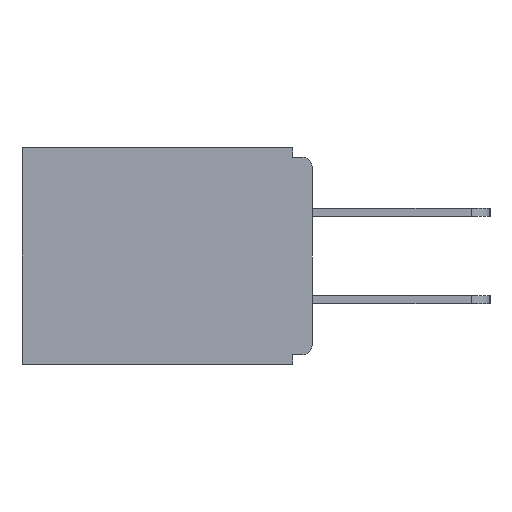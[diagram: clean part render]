
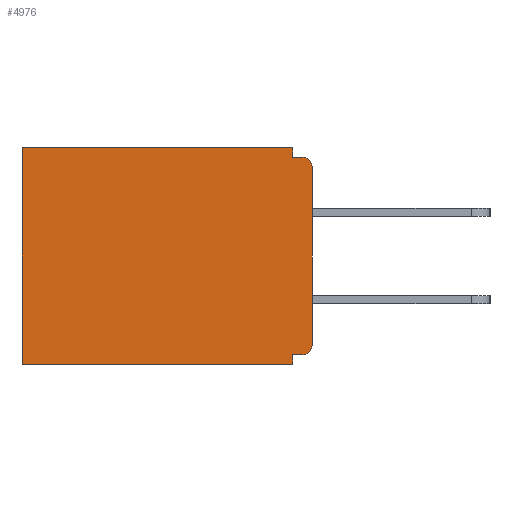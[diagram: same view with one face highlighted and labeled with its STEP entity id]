
A CAD part, left-side view. The second image highlights one B-rep face of the part: STEP entity #4976.
In plain terms, the highlighted planar face has unit normal (-1, 0, 0).
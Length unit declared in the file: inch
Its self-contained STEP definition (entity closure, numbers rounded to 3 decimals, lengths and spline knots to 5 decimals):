
#96 = CARTESIAN_POINT ( 'NONE',  ( 0.298, 0.46, 0. ) ) ;
#584 = ORIENTED_EDGE ( 'NONE', *, *, #10309, .F. ) ;
#746 = VECTOR ( 'NONE', #6360, 39.37008 ) ;
#1071 = CARTESIAN_POINT ( 'NONE',  ( 0.298, 0.031, -0.343 ) ) ;
#1100 = VERTEX_POINT ( 'NONE', #13510 ) ;
#1137 = VECTOR ( 'NONE', #1283, 39.37008 ) ;
#1283 = DIRECTION ( 'NONE',  ( 0., 0., -1. ) ) ;
#1432 = CARTESIAN_POINT ( 'NONE',  ( 0.298, 0., 0. ) ) ;
#1663 = CARTESIAN_POINT ( 'NONE',  ( 0.298, 0., -0.03 ) ) ;
#1769 = ORIENTED_EDGE ( 'NONE', *, *, #7219, .F. ) ;
#2150 = VECTOR ( 'NONE', #5401, 39.37008 ) ;
#2573 = ORIENTED_EDGE ( 'NONE', *, *, #8104, .T. ) ;
#2772 = DIRECTION ( 'NONE',  ( 1., 0., 0. ) ) ;
#2856 = LINE ( 'NONE', #5143, #14362 ) ;
#2864 = VERTEX_POINT ( 'NONE', #1663 ) ;
#2973 = DIRECTION ( 'NONE',  ( 0., 0., -1. ) ) ;
#3009 = DIRECTION ( 'NONE',  ( -1., 0., 0. ) ) ;
#3091 = DIRECTION ( 'NONE',  ( 0., 0., -1. ) ) ;
#3565 = CARTESIAN_POINT ( 'NONE',  ( 0.298, 0.46, -0.343 ) ) ;
#3988 = VECTOR ( 'NONE', #12578, 39.37008 ) ;
#4116 = CARTESIAN_POINT ( 'NONE',  ( 0.298, 0., -0.015 ) ) ;
#4319 = ORIENTED_EDGE ( 'NONE', *, *, #12026, .T. ) ;
#4334 = LINE ( 'NONE', #4500, #5882 ) ;
#4356 = CARTESIAN_POINT ( 'NONE',  ( 0.298, 0., 0. ) ) ;
#4469 = ORIENTED_EDGE ( 'NONE', *, *, #9476, .T. ) ;
#4500 = CARTESIAN_POINT ( 'NONE',  ( 0.298, 0., -0.328 ) ) ;
#4976 = ADVANCED_FACE ( 'NONE', ( #6646 ), #5894, .F. ) ;
#5076 = CARTESIAN_POINT ( 'NONE',  ( 0.298, 0.031, -0.343 ) ) ;
#5143 = CARTESIAN_POINT ( 'NONE',  ( 0.298, 0., 0. ) ) ;
#5272 = EDGE_CURVE ( 'NONE', #5855, #10965, #5939, .T. ) ;
#5401 = DIRECTION ( 'NONE',  ( 0., 0., -1. ) ) ;
#5542 = ORIENTED_EDGE ( 'NONE', *, *, #10551, .F. ) ;
#5549 = CARTESIAN_POINT ( 'NONE',  ( 0.298, 0.015, -0.015 ) ) ;
#5644 = CIRCLE ( 'NONE', #13368, 0.015 ) ;
#5848 = ORIENTED_EDGE ( 'NONE', *, *, #11144, .F. ) ;
#5855 = VERTEX_POINT ( 'NONE', #10150 ) ;
#5882 = VECTOR ( 'NONE', #13455, 39.37008 ) ;
#5894 = PLANE ( 'NONE',  #8700 ) ;
#5939 = LINE ( 'NONE', #10727, #7001 ) ;
#6170 = EDGE_CURVE ( 'NONE', #12209, #12982, #6272, .T. ) ;
#6272 = LINE ( 'NONE', #4356, #7489 ) ;
#6360 = DIRECTION ( 'NONE',  ( 0., -1., 0. ) ) ;
#6646 = FACE_OUTER_BOUND ( 'NONE', #7825, .T. ) ;
#6865 = VERTEX_POINT ( 'NONE', #5549 ) ;
#7001 = VECTOR ( 'NONE', #2973, 39.37008 ) ;
#7097 = DIRECTION ( 'NONE',  ( 0., 0., -1. ) ) ;
#7219 = EDGE_CURVE ( 'NONE', #10965, #10341, #14430, .T. ) ;
#7356 = VERTEX_POINT ( 'NONE', #13682 ) ;
#7489 = VECTOR ( 'NONE', #7721, 39.37008 ) ;
#7721 = DIRECTION ( 'NONE',  ( 0., 1., 0. ) ) ;
#7825 = EDGE_LOOP ( 'NONE', ( #4469, #9227, #5542, #11528, #2573, #1769, #12881, #584, #4319, #5848 ) ) ;
#8104 = EDGE_CURVE ( 'NONE', #12982, #10341, #10113, .T. ) ;
#8196 = AXIS2_PLACEMENT_3D ( 'NONE', #12462, #9392, #7097 ) ;
#8673 = LINE ( 'NONE', #5076, #2150 ) ;
#8700 = AXIS2_PLACEMENT_3D ( 'NONE', #1432, #2772, #13931 ) ;
#9227 = ORIENTED_EDGE ( 'NONE', *, *, #9617, .F. ) ;
#9333 = CIRCLE ( 'NONE', #8196, 0.015 ) ;
#9392 = DIRECTION ( 'NONE',  ( -1., 0., 0. ) ) ;
#9476 = EDGE_CURVE ( 'NONE', #2864, #6865, #5644, .T. ) ;
#9617 = EDGE_CURVE ( 'NONE', #7356, #6865, #12645, .T. ) ;
#9678 = CARTESIAN_POINT ( 'NONE',  ( 0.298, 0.031, 0. ) ) ;
#9746 = CARTESIAN_POINT ( 'NONE',  ( 0.298, 0.015, -0.03 ) ) ;
#10113 = LINE ( 'NONE', #96, #1137 ) ;
#10150 = CARTESIAN_POINT ( 'NONE',  ( 0.298, 0.031, -0.328 ) ) ;
#10226 = VERTEX_POINT ( 'NONE', #13402 ) ;
#10309 = EDGE_CURVE ( 'NONE', #1100, #5855, #4334, .T. ) ;
#10341 = VERTEX_POINT ( 'NONE', #3565 ) ;
#10551 = EDGE_CURVE ( 'NONE', #12209, #7356, #8673, .T. ) ;
#10727 = CARTESIAN_POINT ( 'NONE',  ( 0.298, 0.031, -0.343 ) ) ;
#10965 = VERTEX_POINT ( 'NONE', #1071 ) ;
#11144 = EDGE_CURVE ( 'NONE', #2864, #10226, #2856, .T. ) ;
#11482 = CARTESIAN_POINT ( 'NONE',  ( 0.298, 0., -0.343 ) ) ;
#11528 = ORIENTED_EDGE ( 'NONE', *, *, #6170, .T. ) ;
#12026 = EDGE_CURVE ( 'NONE', #1100, #10226, #9333, .T. ) ;
#12209 = VERTEX_POINT ( 'NONE', #9678 ) ;
#12462 = CARTESIAN_POINT ( 'NONE',  ( 0.298, 0.015, -0.313 ) ) ;
#12578 = DIRECTION ( 'NONE',  ( 0., 1., 0. ) ) ;
#12645 = LINE ( 'NONE', #4116, #746 ) ;
#12877 = CARTESIAN_POINT ( 'NONE',  ( 0.298, 0.46, 0. ) ) ;
#12881 = ORIENTED_EDGE ( 'NONE', *, *, #5272, .F. ) ;
#12982 = VERTEX_POINT ( 'NONE', #12877 ) ;
#13368 = AXIS2_PLACEMENT_3D ( 'NONE', #9746, #3009, #14220 ) ;
#13402 = CARTESIAN_POINT ( 'NONE',  ( 0.298, 0., -0.313 ) ) ;
#13455 = DIRECTION ( 'NONE',  ( 0., 1., 0. ) ) ;
#13510 = CARTESIAN_POINT ( 'NONE',  ( 0.298, 0.015, -0.328 ) ) ;
#13682 = CARTESIAN_POINT ( 'NONE',  ( 0.298, 0.031, -0.015 ) ) ;
#13931 = DIRECTION ( 'NONE',  ( 0., 0., -1. ) ) ;
#14220 = DIRECTION ( 'NONE',  ( 0., 0., -1. ) ) ;
#14362 = VECTOR ( 'NONE', #3091, 39.37008 ) ;
#14430 = LINE ( 'NONE', #11482, #3988 ) ;
